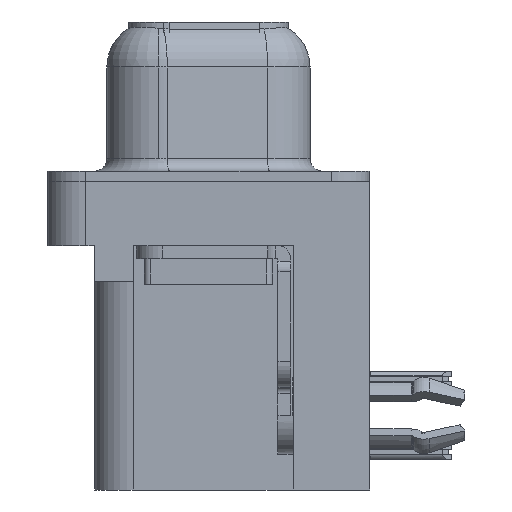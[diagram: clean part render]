
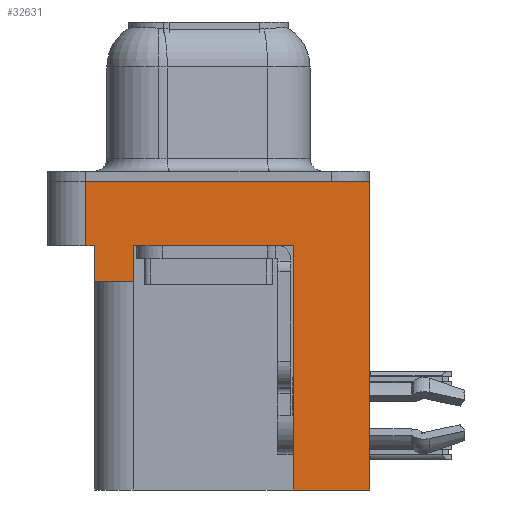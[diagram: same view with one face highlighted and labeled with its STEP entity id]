
A CAD part, left-side view. The second image highlights one B-rep face of the part: STEP entity #32631.
In plain terms, the highlighted planar face has unit normal (-1, 0, 0).
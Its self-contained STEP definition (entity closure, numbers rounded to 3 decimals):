
#260 = VERTEX_POINT ( 'NONE', #17390 ) ;
#1375 = CARTESIAN_POINT ( 'NONE',  ( -3., 4.775, -2.5 ) ) ;
#1527 = VERTEX_POINT ( 'NONE', #27171 ) ;
#1598 = LINE ( 'NONE', #18987, #29989 ) ;
#1642 = VECTOR ( 'NONE', #2067, 1000. ) ;
#1661 = DIRECTION ( 'NONE',  ( 0., 1., 0. ) ) ;
#1946 = LINE ( 'NONE', #27730, #9533 ) ;
#1957 = EDGE_CURVE ( 'NONE', #17714, #2896, #18342, .T. ) ;
#2001 = CARTESIAN_POINT ( 'NONE',  ( -3., -6.275, -2.5 ) ) ;
#2067 = DIRECTION ( 'NONE',  ( 0., 0., 1. ) ) ;
#2300 = CARTESIAN_POINT ( 'NONE',  ( -3., 4.425, -3.9 ) ) ;
#2517 = DIRECTION ( 'NONE',  ( 0., 0., 1. ) ) ;
#2588 = ORIENTED_EDGE ( 'NONE', *, *, #13555, .F. ) ;
#2673 = VERTEX_POINT ( 'NONE', #21900 ) ;
#2896 = VERTEX_POINT ( 'NONE', #14865 ) ;
#3533 = EDGE_CURVE ( 'NONE', #16221, #26454, #8409, .T. ) ;
#3672 = LINE ( 'NONE', #31024, #22400 ) ;
#6396 = DIRECTION ( 'NONE',  ( 0., 0., 1. ) ) ;
#7004 = EDGE_CURVE ( 'NONE', #1527, #16221, #7696, .T. ) ;
#7696 = LINE ( 'NONE', #14335, #16890 ) ;
#8409 = LINE ( 'NONE', #2300, #1642 ) ;
#8454 = EDGE_CURVE ( 'NONE', #21555, #260, #3672, .T. ) ;
#9415 = EDGE_CURVE ( 'NONE', #29839, #26454, #1946, .T. ) ;
#9533 = VECTOR ( 'NONE', #12734, 1000. ) ;
#9592 = DIRECTION ( 'NONE',  ( -1., 0., 0. ) ) ;
#9671 = ORIENTED_EDGE ( 'NONE', *, *, #9415, .T. ) ;
#9722 = DIRECTION ( 'NONE',  ( 0., 1., 0. ) ) ;
#11318 = ORIENTED_EDGE ( 'NONE', *, *, #27073, .F. ) ;
#11808 = CARTESIAN_POINT ( 'NONE',  ( -3., 2.895, -2.5 ) ) ;
#11942 = CARTESIAN_POINT ( 'NONE',  ( -3., 4.425, -2.5 ) ) ;
#12358 = VECTOR ( 'NONE', #14252, 1000. ) ;
#12734 = DIRECTION ( 'NONE',  ( 0., -1., 0. ) ) ;
#13325 = LINE ( 'NONE', #24433, #32902 ) ;
#13555 = EDGE_CURVE ( 'NONE', #28816, #260, #20373, .T. ) ;
#13566 = EDGE_CURVE ( 'NONE', #1527, #17714, #1598, .T. ) ;
#14252 = DIRECTION ( 'NONE',  ( 0., 0., 1. ) ) ;
#14335 = CARTESIAN_POINT ( 'NONE',  ( -3., 4.425, -3.9 ) ) ;
#14865 = CARTESIAN_POINT ( 'NONE',  ( -3., -3.295, -2.5 ) ) ;
#15736 = DIRECTION ( 'NONE',  ( 0., 0., 1. ) ) ;
#16221 = VERTEX_POINT ( 'NONE', #16840 ) ;
#16495 = DIRECTION ( 'NONE',  ( 0., -1., 0. ) ) ;
#16586 = EDGE_CURVE ( 'NONE', #2673, #2896, #30384, .T. ) ;
#16840 = CARTESIAN_POINT ( 'NONE',  ( -3., 4.425, -3.9 ) ) ;
#16890 = VECTOR ( 'NONE', #9722, 1000. ) ;
#17390 = CARTESIAN_POINT ( 'NONE',  ( -3., -6.275, 0. ) ) ;
#17539 = VECTOR ( 'NONE', #16495, 1000. ) ;
#17606 = CARTESIAN_POINT ( 'NONE',  ( -3., -6.275, -12. ) ) ;
#17714 = VERTEX_POINT ( 'NONE', #11808 ) ;
#17802 = CARTESIAN_POINT ( 'NONE',  ( -3., 4.775, -2.5 ) ) ;
#18021 = FACE_OUTER_BOUND ( 'NONE', #24821, .T. ) ;
#18261 = ORIENTED_EDGE ( 'NONE', *, *, #3533, .F. ) ;
#18342 = LINE ( 'NONE', #29026, #17539 ) ;
#18743 = VECTOR ( 'NONE', #26910, 1000. ) ;
#18987 = CARTESIAN_POINT ( 'NONE',  ( -3., 2.895, -3.9 ) ) ;
#19552 = ORIENTED_EDGE ( 'NONE', *, *, #21216, .F. ) ;
#20373 = LINE ( 'NONE', #31826, #18743 ) ;
#21216 = EDGE_CURVE ( 'NONE', #29839, #28816, #22004, .T. ) ;
#21555 = VERTEX_POINT ( 'NONE', #17606 ) ;
#21645 = CARTESIAN_POINT ( 'NONE',  ( -3., -3.295, -12. ) ) ;
#21900 = CARTESIAN_POINT ( 'NONE',  ( -3., -3.295, -12. ) ) ;
#22004 = LINE ( 'NONE', #17802, #31570 ) ;
#22400 = VECTOR ( 'NONE', #15736, 1000. ) ;
#24433 = CARTESIAN_POINT ( 'NONE',  ( -3., -3.295, -12. ) ) ;
#24556 = DIRECTION ( 'NONE',  ( 0., 0., 1. ) ) ;
#24821 = EDGE_LOOP ( 'NONE', ( #2588, #19552, #9671, #18261, #29493, #32856, #27787, #25446, #11318, #30264 ) ) ;
#24876 = PLANE ( 'NONE',  #32591 ) ;
#25446 = ORIENTED_EDGE ( 'NONE', *, *, #16586, .F. ) ;
#25666 = CARTESIAN_POINT ( 'NONE',  ( -3., 4.775, 0. ) ) ;
#26454 = VERTEX_POINT ( 'NONE', #11942 ) ;
#26910 = DIRECTION ( 'NONE',  ( 0., -1., 0. ) ) ;
#27073 = EDGE_CURVE ( 'NONE', #21555, #2673, #13325, .T. ) ;
#27171 = CARTESIAN_POINT ( 'NONE',  ( -3., 2.895, -3.9 ) ) ;
#27730 = CARTESIAN_POINT ( 'NONE',  ( -3., -6.275, -2.5 ) ) ;
#27787 = ORIENTED_EDGE ( 'NONE', *, *, #1957, .T. ) ;
#28816 = VERTEX_POINT ( 'NONE', #25666 ) ;
#29026 = CARTESIAN_POINT ( 'NONE',  ( -3., -6.275, -2.5 ) ) ;
#29493 = ORIENTED_EDGE ( 'NONE', *, *, #7004, .F. ) ;
#29839 = VERTEX_POINT ( 'NONE', #1375 ) ;
#29989 = VECTOR ( 'NONE', #6396, 1000. ) ;
#30264 = ORIENTED_EDGE ( 'NONE', *, *, #8454, .T. ) ;
#30384 = LINE ( 'NONE', #21645, #12358 ) ;
#31024 = CARTESIAN_POINT ( 'NONE',  ( -3., -6.275, -2.5 ) ) ;
#31570 = VECTOR ( 'NONE', #2517, 1000. ) ;
#31826 = CARTESIAN_POINT ( 'NONE',  ( -3., -6.275, 0. ) ) ;
#32591 = AXIS2_PLACEMENT_3D ( 'NONE', #2001, #9592, #24556 ) ;
#32631 = ADVANCED_FACE ( 'NONE', ( #18021 ), #24876, .T. ) ;
#32856 = ORIENTED_EDGE ( 'NONE', *, *, #13566, .T. ) ;
#32902 = VECTOR ( 'NONE', #1661, 1000. ) ;
